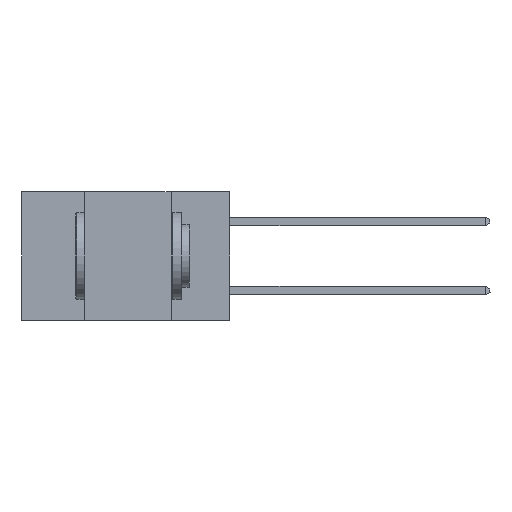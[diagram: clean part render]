
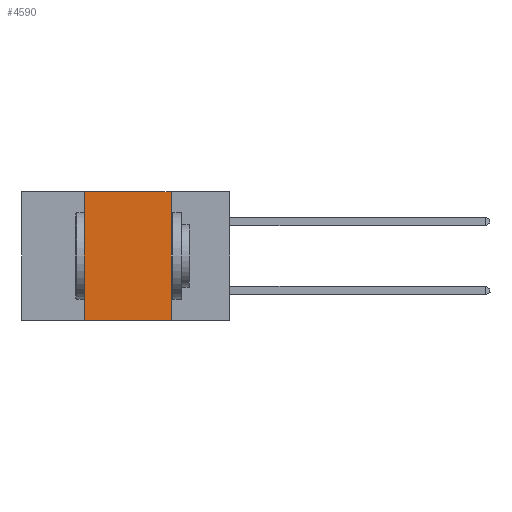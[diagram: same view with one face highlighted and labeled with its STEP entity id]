
A CAD part, left-side view. The second image highlights one B-rep face of the part: STEP entity #4590.
In plain terms, the highlighted planar face has unit normal (-1, 0, 0).
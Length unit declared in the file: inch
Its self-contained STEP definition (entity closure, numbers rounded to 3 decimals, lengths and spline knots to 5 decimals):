
#166 = EDGE_CURVE ( 'NONE', #8837, #17778, #13611, .T. ) ;
#213 = PLANE ( 'NONE',  #16884 ) ;
#821 = CARTESIAN_POINT ( 'NONE',  ( 0., 0.42, 0. ) ) ;
#1808 = DIRECTION ( 'NONE',  ( 0., -1., 0. ) ) ;
#2193 = ORIENTED_EDGE ( 'NONE', *, *, #16470, .F. ) ;
#2787 = CARTESIAN_POINT ( 'NONE',  ( 0., 0.42, -0.37 ) ) ;
#2834 = ORIENTED_EDGE ( 'NONE', *, *, #17896, .T. ) ;
#4112 = EDGE_LOOP ( 'NONE', ( #4215, #2193, #10007, #2834 ) ) ;
#4215 = ORIENTED_EDGE ( 'NONE', *, *, #166, .F. ) ;
#4219 = LINE ( 'NONE', #821, #12811 ) ;
#4590 = ADVANCED_FACE ( 'NONE', ( #17879 ), #213, .F. ) ;
#5005 = DIRECTION ( 'NONE',  ( 0., 0., 1. ) ) ;
#5884 = CARTESIAN_POINT ( 'NONE',  ( 0., 0.6, 0. ) ) ;
#6016 = VECTOR ( 'NONE', #1808, 39.37008 ) ;
#6205 = DIRECTION ( 'NONE',  ( 0., 0., -1. ) ) ;
#8474 = CARTESIAN_POINT ( 'NONE',  ( 0., 0.17, -0.37 ) ) ;
#8607 = CARTESIAN_POINT ( 'NONE',  ( 0., 0.17, 0. ) ) ;
#8837 = VERTEX_POINT ( 'NONE', #16873 ) ;
#10003 = DIRECTION ( 'NONE',  ( 0., 0., -1. ) ) ;
#10007 = ORIENTED_EDGE ( 'NONE', *, *, #17967, .F. ) ;
#10063 = DIRECTION ( 'NONE',  ( 1., 0., 0. ) ) ;
#10904 = CARTESIAN_POINT ( 'NONE',  ( 0., 0.42, 0. ) ) ;
#11518 = LINE ( 'NONE', #11685, #6016 ) ;
#11685 = CARTESIAN_POINT ( 'NONE',  ( 0., 0.6, 0. ) ) ;
#11840 = DIRECTION ( 'NONE',  ( 0., -1., 0. ) ) ;
#12388 = VECTOR ( 'NONE', #11840, 39.37008 ) ;
#12811 = VECTOR ( 'NONE', #5005, 39.37008 ) ;
#13611 = LINE ( 'NONE', #8607, #15378 ) ;
#14612 = CARTESIAN_POINT ( 'NONE',  ( 0., 0.6, -0.37 ) ) ;
#15378 = VECTOR ( 'NONE', #10003, 39.37008 ) ;
#15729 = VERTEX_POINT ( 'NONE', #2787 ) ;
#16126 = LINE ( 'NONE', #14612, #12388 ) ;
#16470 = EDGE_CURVE ( 'NONE', #18251, #8837, #11518, .T. ) ;
#16873 = CARTESIAN_POINT ( 'NONE',  ( 0., 0.17, 0. ) ) ;
#16884 = AXIS2_PLACEMENT_3D ( 'NONE', #5884, #10063, #6205 ) ;
#17778 = VERTEX_POINT ( 'NONE', #8474 ) ;
#17879 = FACE_OUTER_BOUND ( 'NONE', #4112, .T. ) ;
#17896 = EDGE_CURVE ( 'NONE', #15729, #17778, #16126, .T. ) ;
#17967 = EDGE_CURVE ( 'NONE', #15729, #18251, #4219, .T. ) ;
#18251 = VERTEX_POINT ( 'NONE', #10904 ) ;
